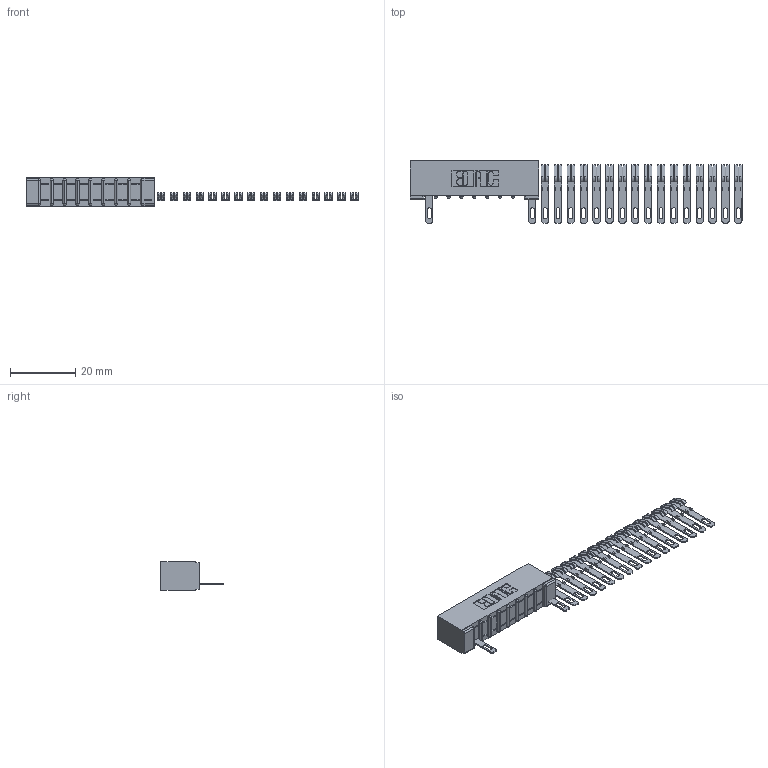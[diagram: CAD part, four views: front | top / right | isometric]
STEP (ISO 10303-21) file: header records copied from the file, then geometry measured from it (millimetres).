
FILE_DESCRIPTION (( 'STEP AP203' ), '1' );
FILE_NAME ('357-025-505-101.STEP', '2018-08-09T01:28:27', ( '' ), ( '' ), 'SwSTEP 2.0', 'SolidWorks 2016', '' );
FILE_SCHEMA (( 'CONFIG_CONTROL_DESIGN' ));
Length unit declared in the file: inch
Products named in the file (3): 357-025-505-101; 307 Part_No Mounting Lugs; 307-290-001_505
Assembly tree (19 placements, depth 2):
  357-025-505-101
    307 Part_No Mounting Lugs
    307-290-001_505  x18
Bounding box: 102.15 x 19.18 x 8.71 mm (x, y, z)
Volume: 2901.5 mm3; surface area: 5309.7 mm2
Topology: 19 solids, 19 shells, 927 faces, 2575 edges, 1666 vertices
Faces by surface type: plane 594, cylinder 315, sphere 18
Entity records: 11066 total; most frequent: CARTESIAN_POINT 1806, DIRECTION 1787, ORIENTED_EDGE 1782, EDGE_CURVE 891, VECTOR 669, LINE 669, VERTEX_POINT 578, AXIS2_PLACEMENT_3D 559
